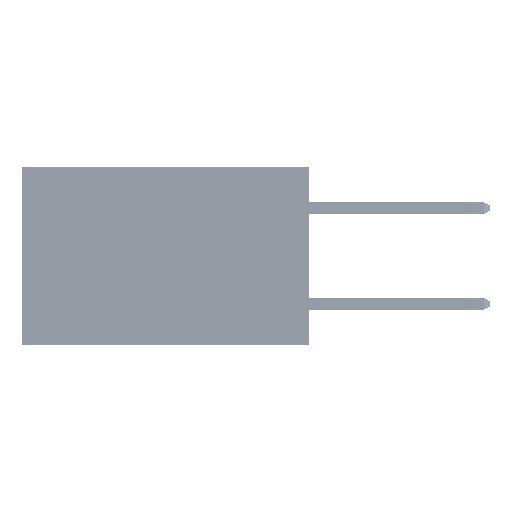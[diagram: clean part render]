
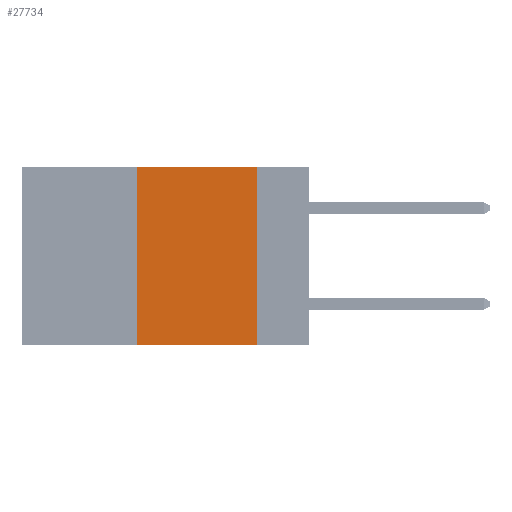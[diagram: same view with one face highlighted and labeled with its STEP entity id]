
A CAD part, left-side view. The second image highlights one B-rep face of the part: STEP entity #27734.
In plain terms, the highlighted planar face has unit normal (-1, 0, 0).
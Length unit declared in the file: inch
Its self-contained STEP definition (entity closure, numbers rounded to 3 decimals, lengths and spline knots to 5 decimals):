
#5156 = CARTESIAN_POINT ( 'NONE',  ( 0., 0.11, -0.37 ) ) ;
#6051 = LINE ( 'NONE', #39333, #25715 ) ;
#6715 = AXIS2_PLACEMENT_3D ( 'NONE', #23623, #27196, #20029 ) ;
#8845 = VECTOR ( 'NONE', #25566, 39.37008 ) ;
#10713 = EDGE_CURVE ( 'NONE', #11031, #36711, #42126, .T. ) ;
#11031 = VERTEX_POINT ( 'NONE', #25218 ) ;
#13777 = CARTESIAN_POINT ( 'NONE',  ( 0., 0.6, -0.37 ) ) ;
#16066 = PLANE ( 'NONE',  #6715 ) ;
#16331 = DIRECTION ( 'NONE',  ( 0., 0., -1. ) ) ;
#17084 = ORIENTED_EDGE ( 'NONE', *, *, #44513, .F. ) ;
#20029 = DIRECTION ( 'NONE',  ( 0., 0., -1. ) ) ;
#20155 = VECTOR ( 'NONE', #16331, 39.37008 ) ;
#23623 = CARTESIAN_POINT ( 'NONE',  ( 0., 0.6, 0. ) ) ;
#23713 = CARTESIAN_POINT ( 'NONE',  ( 0., 0.11, 0. ) ) ;
#23812 = DIRECTION ( 'NONE',  ( 0., -1., 0. ) ) ;
#25218 = CARTESIAN_POINT ( 'NONE',  ( 0., 0.11, 0. ) ) ;
#25566 = DIRECTION ( 'NONE',  ( 0., -1., 0. ) ) ;
#25715 = VECTOR ( 'NONE', #23812, 39.37008 ) ;
#26761 = EDGE_CURVE ( 'NONE', #35834, #36711, #43685, .T. ) ;
#27196 = DIRECTION ( 'NONE',  ( 1., 0., 0. ) ) ;
#27446 = LINE ( 'NONE', #49032, #41513 ) ;
#27734 = ADVANCED_FACE ( 'NONE', ( #40655 ), #16066, .F. ) ;
#34565 = EDGE_CURVE ( 'NONE', #35834, #44412, #27446, .T. ) ;
#35834 = VERTEX_POINT ( 'NONE', #43008 ) ;
#36711 = VERTEX_POINT ( 'NONE', #5156 ) ;
#37631 = ORIENTED_EDGE ( 'NONE', *, *, #10713, .F. ) ;
#39333 = CARTESIAN_POINT ( 'NONE',  ( 0., 0.6, 0. ) ) ;
#40655 = FACE_OUTER_BOUND ( 'NONE', #45886, .T. ) ;
#41513 = VECTOR ( 'NONE', #45233, 39.37008 ) ;
#42126 = LINE ( 'NONE', #23713, #20155 ) ;
#43008 = CARTESIAN_POINT ( 'NONE',  ( 0., 0.36, -0.37 ) ) ;
#43685 = LINE ( 'NONE', #13777, #8845 ) ;
#44412 = VERTEX_POINT ( 'NONE', #46495 ) ;
#44513 = EDGE_CURVE ( 'NONE', #44412, #11031, #6051, .T. ) ;
#45061 = ORIENTED_EDGE ( 'NONE', *, *, #26761, .T. ) ;
#45233 = DIRECTION ( 'NONE',  ( 0., 0., 1. ) ) ;
#45886 = EDGE_LOOP ( 'NONE', ( #37631, #17084, #46998, #45061 ) ) ;
#46495 = CARTESIAN_POINT ( 'NONE',  ( 0., 0.36, 0. ) ) ;
#46998 = ORIENTED_EDGE ( 'NONE', *, *, #34565, .F. ) ;
#49032 = CARTESIAN_POINT ( 'NONE',  ( 0., 0.36, 0. ) ) ;
